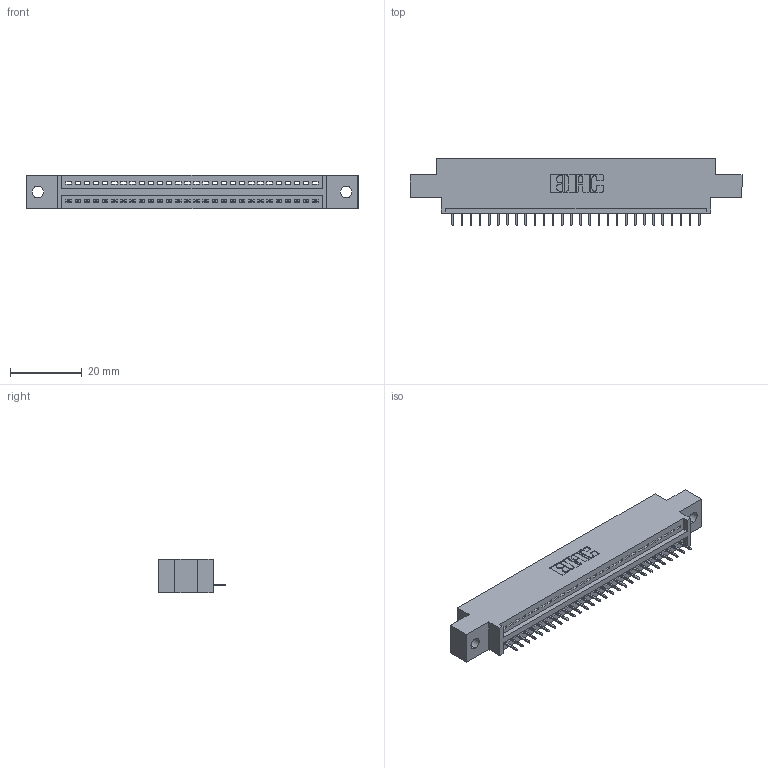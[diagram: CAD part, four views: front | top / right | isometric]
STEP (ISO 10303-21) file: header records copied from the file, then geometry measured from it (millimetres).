
FILE_DESCRIPTION (( 'STEP AP203' ), '1' );
FILE_NAME ('845-028-525-602.STEP', '2020-09-22T23:30:10', ( '' ), ( '' ), 'SwSTEP 2.0', 'SolidWorks 2020', '' );
FILE_SCHEMA (( 'CONFIG_CONTROL_DESIGN' ));
Length unit declared in the file: inch
Products named in the file (3): 845 Part_0.170 Offset - 0.128 Dia; 845-028-525-602; 345-292-001_345-293-125
Assembly tree (29 placements, depth 2):
  845-028-525-602
    845 Part_0.170 Offset - 0.128 Dia
    345-292-001_345-293-125  x28
Bounding box: 92.33 x 18.72 x 9.4 mm (x, y, z)
Volume: 8390.4 mm3; surface area: 10433.7 mm2
Topology: 29 solids, 29 shells, 1866 faces, 5393 edges, 3482 vertices
Faces by surface type: plane 1372, cylinder 494
Entity records: 23167 total; most frequent: CARTESIAN_POINT 4020, ORIENTED_EDGE 3982, DIRECTION 3531, EDGE_CURVE 1991, VECTOR 1751, LINE 1751, VERTEX_POINT 1322, AXIS2_PLACEMENT_3D 890
